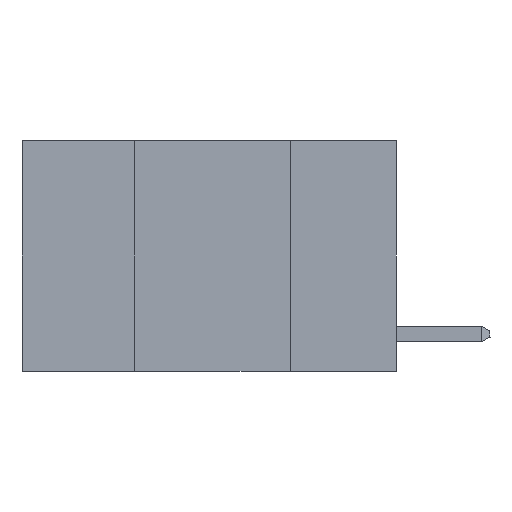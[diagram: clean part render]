
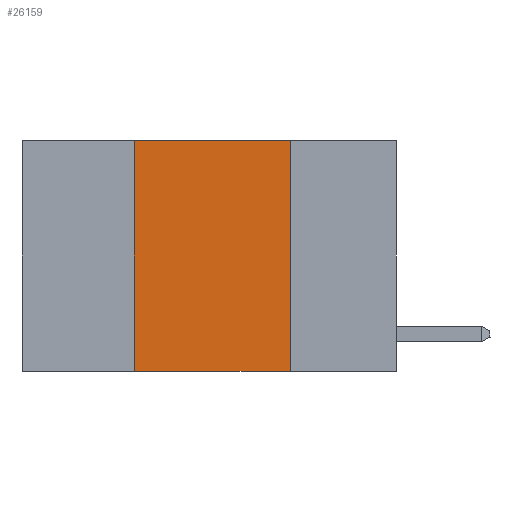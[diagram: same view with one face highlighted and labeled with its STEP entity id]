
A CAD part, left-side view. The second image highlights one B-rep face of the part: STEP entity #26159.
In plain terms, the highlighted planar face has unit normal (-1, 0, 0).
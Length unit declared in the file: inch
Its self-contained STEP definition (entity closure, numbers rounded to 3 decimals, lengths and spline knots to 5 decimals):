
#703 = VECTOR ( 'NONE', #17257, 39.37008 ) ;
#1760 = ORIENTED_EDGE ( 'NONE', *, *, #17235, .F. ) ;
#2577 = CARTESIAN_POINT ( 'NONE',  ( 0., 0.42, 0. ) ) ;
#4454 = CARTESIAN_POINT ( 'NONE',  ( 0., 0.42, 0. ) ) ;
#4914 = EDGE_CURVE ( 'NONE', #8146, #21563, #6873, .T. ) ;
#5242 = CARTESIAN_POINT ( 'NONE',  ( 0., 0.17, 0. ) ) ;
#5434 = CARTESIAN_POINT ( 'NONE',  ( 0., 0.17, 0. ) ) ;
#5690 = FACE_OUTER_BOUND ( 'NONE', #25840, .T. ) ;
#5826 = CARTESIAN_POINT ( 'NONE',  ( 0., 0.6, 0. ) ) ;
#5934 = DIRECTION ( 'NONE',  ( 0., 0., -1. ) ) ;
#6529 = ORIENTED_EDGE ( 'NONE', *, *, #30099, .F. ) ;
#6608 = CARTESIAN_POINT ( 'NONE',  ( 0., 0.6, -0.37 ) ) ;
#6842 = DIRECTION ( 'NONE',  ( 0., 0., 1. ) ) ;
#6873 = LINE ( 'NONE', #13489, #25143 ) ;
#8146 = VERTEX_POINT ( 'NONE', #2577 ) ;
#9804 = VECTOR ( 'NONE', #16241, 39.37008 ) ;
#11042 = ORIENTED_EDGE ( 'NONE', *, *, #30694, .T. ) ;
#12153 = ORIENTED_EDGE ( 'NONE', *, *, #4914, .F. ) ;
#13302 = VERTEX_POINT ( 'NONE', #15688 ) ;
#13410 = LINE ( 'NONE', #5242, #703 ) ;
#13489 = CARTESIAN_POINT ( 'NONE',  ( 0., 0.6, 0. ) ) ;
#15473 = LINE ( 'NONE', #4454, #27333 ) ;
#15688 = CARTESIAN_POINT ( 'NONE',  ( 0., 0.17, -0.37 ) ) ;
#16160 = LINE ( 'NONE', #6608, #9804 ) ;
#16241 = DIRECTION ( 'NONE',  ( 0., -1., 0. ) ) ;
#17235 = EDGE_CURVE ( 'NONE', #21563, #13302, #13410, .T. ) ;
#17257 = DIRECTION ( 'NONE',  ( 0., 0., -1. ) ) ;
#17823 = PLANE ( 'NONE',  #24267 ) ;
#20213 = DIRECTION ( 'NONE',  ( 1., 0., 0. ) ) ;
#20252 = CARTESIAN_POINT ( 'NONE',  ( 0., 0.42, -0.37 ) ) ;
#21563 = VERTEX_POINT ( 'NONE', #5434 ) ;
#23125 = VERTEX_POINT ( 'NONE', #20252 ) ;
#24267 = AXIS2_PLACEMENT_3D ( 'NONE', #5826, #20213, #5934 ) ;
#25143 = VECTOR ( 'NONE', #25321, 39.37008 ) ;
#25321 = DIRECTION ( 'NONE',  ( 0., -1., 0. ) ) ;
#25840 = EDGE_LOOP ( 'NONE', ( #1760, #12153, #6529, #11042 ) ) ;
#26159 = ADVANCED_FACE ( 'NONE', ( #5690 ), #17823, .F. ) ;
#27333 = VECTOR ( 'NONE', #6842, 39.37008 ) ;
#30099 = EDGE_CURVE ( 'NONE', #23125, #8146, #15473, .T. ) ;
#30694 = EDGE_CURVE ( 'NONE', #23125, #13302, #16160, .T. ) ;
